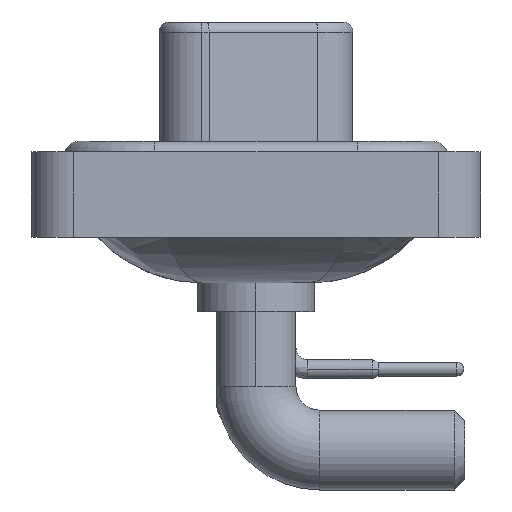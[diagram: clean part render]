
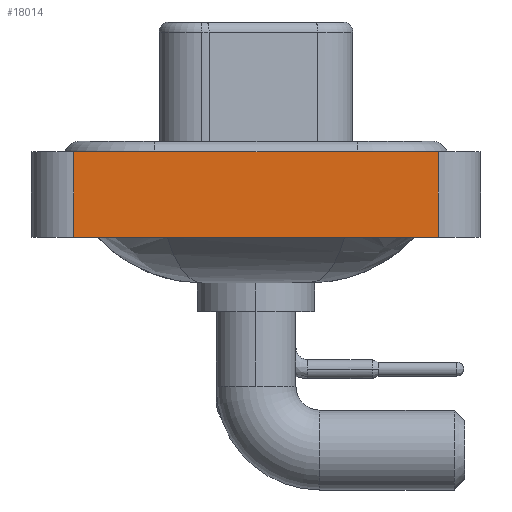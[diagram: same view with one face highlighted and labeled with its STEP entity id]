
A CAD part, left-side view. The second image highlights one B-rep face of the part: STEP entity #18014.
In plain terms, the highlighted planar face has unit normal (-1, 0, 0).
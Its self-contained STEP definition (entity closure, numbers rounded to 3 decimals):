
#214 = FACE_OUTER_BOUND ( 'NONE', #7342, .T. ) ;
#529 = LINE ( 'NONE', #20515, #12667 ) ;
#1428 = EDGE_CURVE ( 'NONE', #12031, #1744, #4752, .T. ) ;
#1744 = VERTEX_POINT ( 'NONE', #26044 ) ;
#2208 = DIRECTION ( 'NONE',  ( 0., 0., 1. ) ) ;
#2528 = CARTESIAN_POINT ( 'NONE',  ( -7.35, 8.55, -3.6 ) ) ;
#2749 = ORIENTED_EDGE ( 'NONE', *, *, #15960, .T. ) ;
#3509 = AXIS2_PLACEMENT_3D ( 'NONE', #26162, #10288, #2208 ) ;
#4061 = CARTESIAN_POINT ( 'NONE',  ( -7.35, -8.55, 0.4 ) ) ;
#4752 = LINE ( 'NONE', #14919, #13427 ) ;
#5209 = DIRECTION ( 'NONE',  ( 0., 0., 1. ) ) ;
#7342 = EDGE_LOOP ( 'NONE', ( #22686, #16074, #17462, #2749 ) ) ;
#8950 = EDGE_CURVE ( 'NONE', #12797, #14253, #15826, .T. ) ;
#10033 = PLANE ( 'NONE',  #3509 ) ;
#10281 = DIRECTION ( 'NONE',  ( 0., -1., 0. ) ) ;
#10288 = DIRECTION ( 'NONE',  ( -1., 0., 0. ) ) ;
#10562 = VECTOR ( 'NONE', #10281, 1000. ) ;
#12031 = VERTEX_POINT ( 'NONE', #17658 ) ;
#12667 = VECTOR ( 'NONE', #23166, 1000. ) ;
#12797 = VERTEX_POINT ( 'NONE', #2528 ) ;
#13427 = VECTOR ( 'NONE', #24882, 1000. ) ;
#14253 = VERTEX_POINT ( 'NONE', #18254 ) ;
#14919 = CARTESIAN_POINT ( 'NONE',  ( -7.35, -8.55, -3.6 ) ) ;
#15826 = LINE ( 'NONE', #22191, #17188 ) ;
#15960 = EDGE_CURVE ( 'NONE', #12797, #12031, #529, .T. ) ;
#16074 = ORIENTED_EDGE ( 'NONE', *, *, #16303, .F. ) ;
#16303 = EDGE_CURVE ( 'NONE', #14253, #1744, #22180, .T. ) ;
#17188 = VECTOR ( 'NONE', #5209, 1000. ) ;
#17462 = ORIENTED_EDGE ( 'NONE', *, *, #8950, .F. ) ;
#17658 = CARTESIAN_POINT ( 'NONE',  ( -7.35, -8.55, -3.6 ) ) ;
#18014 = ADVANCED_FACE ( 'NONE', ( #214 ), #10033, .T. ) ;
#18254 = CARTESIAN_POINT ( 'NONE',  ( -7.35, 8.55, 0.4 ) ) ;
#20515 = CARTESIAN_POINT ( 'NONE',  ( -7.35, -8.55, -3.6 ) ) ;
#22180 = LINE ( 'NONE', #4061, #10562 ) ;
#22191 = CARTESIAN_POINT ( 'NONE',  ( -7.35, 8.55, -3.6 ) ) ;
#22686 = ORIENTED_EDGE ( 'NONE', *, *, #1428, .T. ) ;
#23166 = DIRECTION ( 'NONE',  ( 0., -1., 0. ) ) ;
#24882 = DIRECTION ( 'NONE',  ( 0., 0., 1. ) ) ;
#26044 = CARTESIAN_POINT ( 'NONE',  ( -7.35, -8.55, 0.4 ) ) ;
#26162 = CARTESIAN_POINT ( 'NONE',  ( -7.35, -8.55, -3.6 ) ) ;
